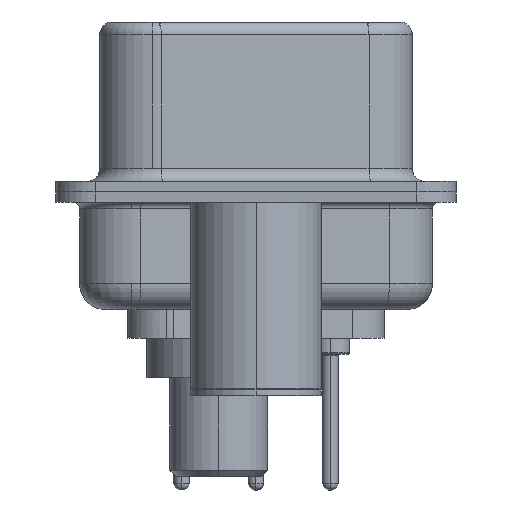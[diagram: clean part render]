
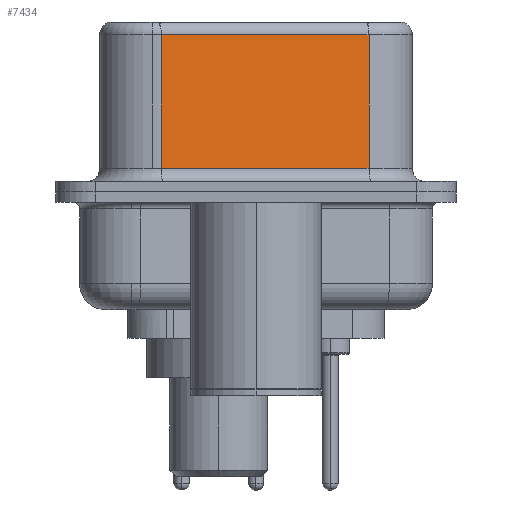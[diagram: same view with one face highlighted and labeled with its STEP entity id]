
A CAD part, left-side view. The second image highlights one B-rep face of the part: STEP entity #7434.
In plain terms, the highlighted planar face has unit normal (-0.985, -0.174, 0).
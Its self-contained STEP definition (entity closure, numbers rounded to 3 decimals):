
#2913 = VERTEX_POINT ( 'NONE', #12766 ) ;
#2954 = VECTOR ( 'NONE', #15888, 1000. ) ;
#3171 = EDGE_CURVE ( 'NONE', #23964, #25092, #15607, .T. ) ;
#4221 = DIRECTION ( 'NONE',  ( 0., 0., -1. ) ) ;
#6699 = VECTOR ( 'NONE', #4221, 1000. ) ;
#7154 = DIRECTION ( 'NONE',  ( -0.174, 0.985, 0. ) ) ;
#7240 = DIRECTION ( 'NONE',  ( 0.985, 0.174, 0. ) ) ;
#7434 = ADVANCED_FACE ( 'NONE', ( #10552 ), #26246, .F. ) ;
#9561 = CARTESIAN_POINT ( 'NONE',  ( 5.132, -4.322, 6.52 ) ) ;
#10552 = FACE_OUTER_BOUND ( 'NONE', #12268, .T. ) ;
#10578 = ORIENTED_EDGE ( 'NONE', *, *, #17232, .F. ) ;
#10669 = CARTESIAN_POINT ( 'NONE',  ( 5.132, -4.322, 0.9 ) ) ;
#12069 = VECTOR ( 'NONE', #19180, 1000. ) ;
#12268 = EDGE_LOOP ( 'NONE', ( #10578, #13798, #23051, #24512 ) ) ;
#12766 = CARTESIAN_POINT ( 'NONE',  ( 3.73, 3.628, 6.02 ) ) ;
#13493 = LINE ( 'NONE', #14504, #6699 ) ;
#13798 = ORIENTED_EDGE ( 'NONE', *, *, #21562, .T. ) ;
#14504 = CARTESIAN_POINT ( 'NONE',  ( 3.73, 3.628, 6.52 ) ) ;
#15414 = CARTESIAN_POINT ( 'NONE',  ( 5.132, -4.322, 0.9 ) ) ;
#15607 = LINE ( 'NONE', #15414, #12069 ) ;
#15888 = DIRECTION ( 'NONE',  ( 0., 0., -1. ) ) ;
#16667 = VECTOR ( 'NONE', #25885, 1000. ) ;
#17232 = EDGE_CURVE ( 'NONE', #25686, #25092, #19491, .T. ) ;
#19180 = DIRECTION ( 'NONE',  ( 0.174, -0.985, 0. ) ) ;
#19491 = LINE ( 'NONE', #20082, #2954 ) ;
#20082 = CARTESIAN_POINT ( 'NONE',  ( 5.132, -4.322, 6.52 ) ) ;
#20113 = CARTESIAN_POINT ( 'NONE',  ( 3.73, 3.628, 0.9 ) ) ;
#20165 = EDGE_CURVE ( 'NONE', #2913, #23964, #13493, .T. ) ;
#20826 = AXIS2_PLACEMENT_3D ( 'NONE', #9561, #7240, #7154 ) ;
#21562 = EDGE_CURVE ( 'NONE', #25686, #2913, #22229, .T. ) ;
#22229 = LINE ( 'NONE', #23806, #16667 ) ;
#23051 = ORIENTED_EDGE ( 'NONE', *, *, #20165, .T. ) ;
#23093 = CARTESIAN_POINT ( 'NONE',  ( 5.132, -4.322, 6.02 ) ) ;
#23806 = CARTESIAN_POINT ( 'NONE',  ( 5.132, -4.322, 6.02 ) ) ;
#23964 = VERTEX_POINT ( 'NONE', #20113 ) ;
#24512 = ORIENTED_EDGE ( 'NONE', *, *, #3171, .T. ) ;
#25092 = VERTEX_POINT ( 'NONE', #10669 ) ;
#25686 = VERTEX_POINT ( 'NONE', #23093 ) ;
#25885 = DIRECTION ( 'NONE',  ( -0.174, 0.985, 0. ) ) ;
#26246 = PLANE ( 'NONE',  #20826 ) ;
